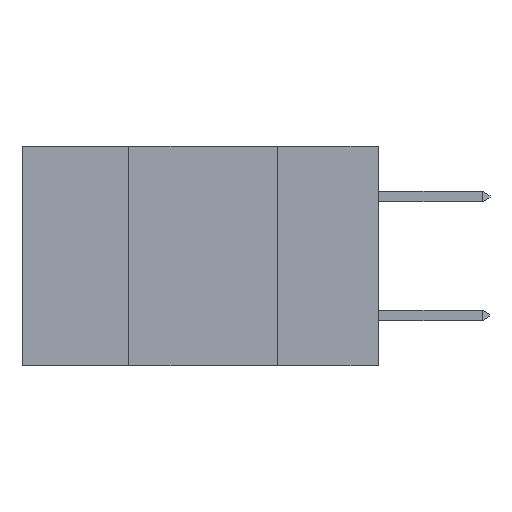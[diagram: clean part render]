
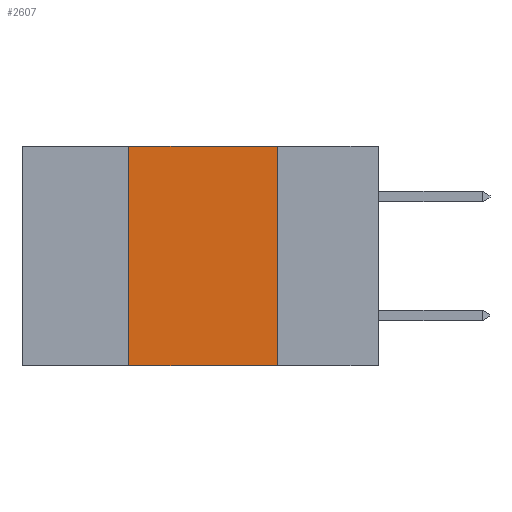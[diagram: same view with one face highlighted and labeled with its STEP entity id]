
A CAD part, left-side view. The second image highlights one B-rep face of the part: STEP entity #2607.
In plain terms, the highlighted planar face has unit normal (-1, 0, 0).
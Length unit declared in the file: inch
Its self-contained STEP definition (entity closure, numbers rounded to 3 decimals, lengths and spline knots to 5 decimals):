
#1004 = CARTESIAN_POINT ( 'NONE',  ( 0., 0.17, 0. ) ) ;
#1382 = EDGE_CURVE ( 'NONE', #6823, #17077, #19758, .T. ) ;
#1673 = EDGE_CURVE ( 'NONE', #17077, #18713, #17473, .T. ) ;
#2607 = ADVANCED_FACE ( 'NONE', ( #15417 ), #11907, .F. ) ;
#2955 = VECTOR ( 'NONE', #15156, 39.37008 ) ;
#3095 = DIRECTION ( 'NONE',  ( 0., -1., 0. ) ) ;
#4608 = AXIS2_PLACEMENT_3D ( 'NONE', #11883, #11970, #11956 ) ;
#5888 = VECTOR ( 'NONE', #3095, 39.37008 ) ;
#6823 = VERTEX_POINT ( 'NONE', #18964 ) ;
#6900 = DIRECTION ( 'NONE',  ( 0., 0., 1. ) ) ;
#7011 = CARTESIAN_POINT ( 'NONE',  ( 0., 0.42, 0. ) ) ;
#7035 = VECTOR ( 'NONE', #6900, 39.37008 ) ;
#7125 = LINE ( 'NONE', #7193, #2955 ) ;
#7193 = CARTESIAN_POINT ( 'NONE',  ( 0., 0.17, 0. ) ) ;
#7222 = ORIENTED_EDGE ( 'NONE', *, *, #15075, .F. ) ;
#9439 = VECTOR ( 'NONE', #19369, 39.37008 ) ;
#9510 = LINE ( 'NONE', #12522, #5888 ) ;
#9955 = VERTEX_POINT ( 'NONE', #19929 ) ;
#11085 = ORIENTED_EDGE ( 'NONE', *, *, #12146, .T. ) ;
#11883 = CARTESIAN_POINT ( 'NONE',  ( 0., 0.6, 0. ) ) ;
#11907 = PLANE ( 'NONE',  #4608 ) ;
#11956 = DIRECTION ( 'NONE',  ( 0., 0., -1. ) ) ;
#11970 = DIRECTION ( 'NONE',  ( 1., 0., 0. ) ) ;
#12146 = EDGE_CURVE ( 'NONE', #6823, #9955, #9510, .T. ) ;
#12522 = CARTESIAN_POINT ( 'NONE',  ( 0., 0.6, -0.37 ) ) ;
#14611 = EDGE_LOOP ( 'NONE', ( #7222, #19636, #19198, #11085 ) ) ;
#15075 = EDGE_CURVE ( 'NONE', #18713, #9955, #7125, .T. ) ;
#15156 = DIRECTION ( 'NONE',  ( 0., 0., -1. ) ) ;
#15417 = FACE_OUTER_BOUND ( 'NONE', #14611, .T. ) ;
#17077 = VERTEX_POINT ( 'NONE', #17619 ) ;
#17473 = LINE ( 'NONE', #19389, #9439 ) ;
#17619 = CARTESIAN_POINT ( 'NONE',  ( 0., 0.42, 0. ) ) ;
#18713 = VERTEX_POINT ( 'NONE', #1004 ) ;
#18964 = CARTESIAN_POINT ( 'NONE',  ( 0., 0.42, -0.37 ) ) ;
#19198 = ORIENTED_EDGE ( 'NONE', *, *, #1382, .F. ) ;
#19369 = DIRECTION ( 'NONE',  ( 0., -1., 0. ) ) ;
#19389 = CARTESIAN_POINT ( 'NONE',  ( 0., 0.6, 0. ) ) ;
#19636 = ORIENTED_EDGE ( 'NONE', *, *, #1673, .F. ) ;
#19758 = LINE ( 'NONE', #7011, #7035 ) ;
#19929 = CARTESIAN_POINT ( 'NONE',  ( 0., 0.17, -0.37 ) ) ;
